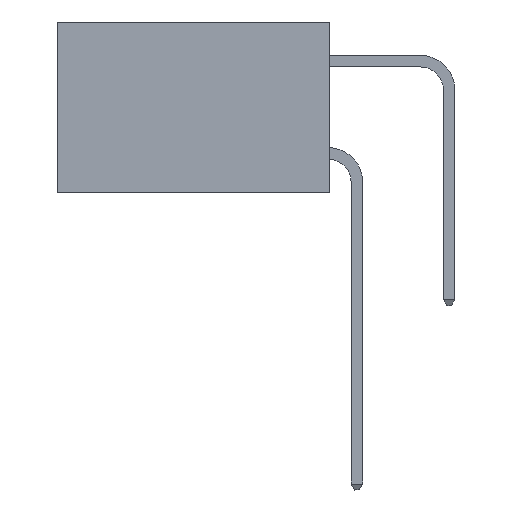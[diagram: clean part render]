
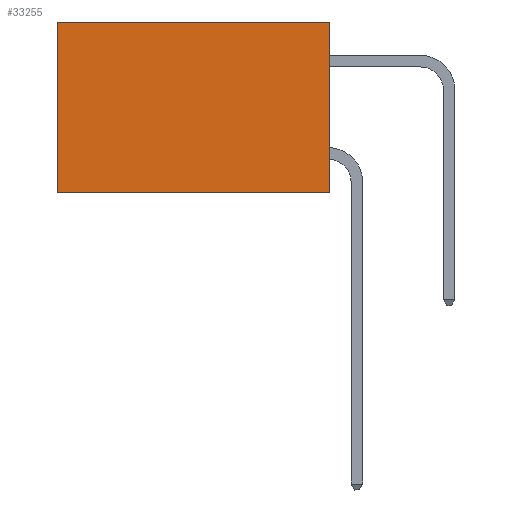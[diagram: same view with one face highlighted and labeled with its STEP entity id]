
A CAD part, left-side view. The second image highlights one B-rep face of the part: STEP entity #33255.
In plain terms, the highlighted planar face has unit normal (-1, 0, 0).
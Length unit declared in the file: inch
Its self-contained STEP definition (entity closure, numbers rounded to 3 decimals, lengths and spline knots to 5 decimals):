
#135 = VERTEX_POINT ( 'NONE', #32950 ) ;
#450 = CARTESIAN_POINT ( 'NONE',  ( 0.277, 0., -0.37 ) ) ;
#1394 = VERTEX_POINT ( 'NONE', #10452 ) ;
#1442 = LINE ( 'NONE', #12510, #14747 ) ;
#3432 = VECTOR ( 'NONE', #26113, 39.37008 ) ;
#4975 = DIRECTION ( 'NONE',  ( 0., 1., 0. ) ) ;
#5018 = CARTESIAN_POINT ( 'NONE',  ( 0.277, 0., 0. ) ) ;
#5337 = VECTOR ( 'NONE', #4975, 39.37008 ) ;
#6536 = AXIS2_PLACEMENT_3D ( 'NONE', #27208, #11435, #29793 ) ;
#8785 = PLANE ( 'NONE',  #6536 ) ;
#10452 = CARTESIAN_POINT ( 'NONE',  ( 0.277, 0.59, 0. ) ) ;
#10482 = LINE ( 'NONE', #5018, #3432 ) ;
#11340 = EDGE_LOOP ( 'NONE', ( #20989, #29996, #16939, #14058 ) ) ;
#11435 = DIRECTION ( 'NONE',  ( 1., 0., 0. ) ) ;
#11553 = LINE ( 'NONE', #20823, #5337 ) ;
#12417 = LINE ( 'NONE', #450, #24754 ) ;
#12510 = CARTESIAN_POINT ( 'NONE',  ( 0.277, 0.59, -0.37 ) ) ;
#14058 = ORIENTED_EDGE ( 'NONE', *, *, #32260, .T. ) ;
#14747 = VECTOR ( 'NONE', #33482, 39.37008 ) ;
#15059 = CARTESIAN_POINT ( 'NONE',  ( 0.277, 0.59, -0.37 ) ) ;
#15633 = VERTEX_POINT ( 'NONE', #15059 ) ;
#16939 = ORIENTED_EDGE ( 'NONE', *, *, #21827, .F. ) ;
#20823 = CARTESIAN_POINT ( 'NONE',  ( 0.277, 0., -0.37 ) ) ;
#20989 = ORIENTED_EDGE ( 'NONE', *, *, #30756, .T. ) ;
#21674 = DIRECTION ( 'NONE',  ( 0., 0., -1. ) ) ;
#21827 = EDGE_CURVE ( 'NONE', #135, #24826, #12417, .T. ) ;
#22277 = EDGE_CURVE ( 'NONE', #24826, #15633, #11553, .T. ) ;
#24754 = VECTOR ( 'NONE', #21674, 39.37008 ) ;
#24826 = VERTEX_POINT ( 'NONE', #30102 ) ;
#26113 = DIRECTION ( 'NONE',  ( 0., 1., 0. ) ) ;
#27208 = CARTESIAN_POINT ( 'NONE',  ( 0.277, 0., -0.37 ) ) ;
#29793 = DIRECTION ( 'NONE',  ( 0., 0., -1. ) ) ;
#29996 = ORIENTED_EDGE ( 'NONE', *, *, #22277, .F. ) ;
#30073 = FACE_OUTER_BOUND ( 'NONE', #11340, .T. ) ;
#30102 = CARTESIAN_POINT ( 'NONE',  ( 0.277, 0., -0.37 ) ) ;
#30756 = EDGE_CURVE ( 'NONE', #1394, #15633, #1442, .T. ) ;
#32260 = EDGE_CURVE ( 'NONE', #135, #1394, #10482, .T. ) ;
#32950 = CARTESIAN_POINT ( 'NONE',  ( 0.277, 0., 0. ) ) ;
#33255 = ADVANCED_FACE ( 'NONE', ( #30073 ), #8785, .F. ) ;
#33482 = DIRECTION ( 'NONE',  ( 0., 0., -1. ) ) ;
